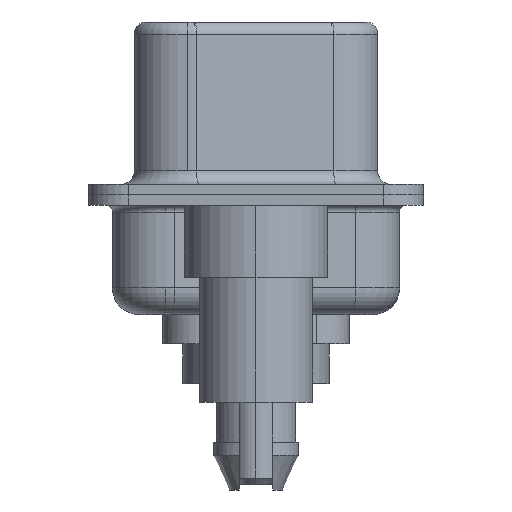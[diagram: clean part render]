
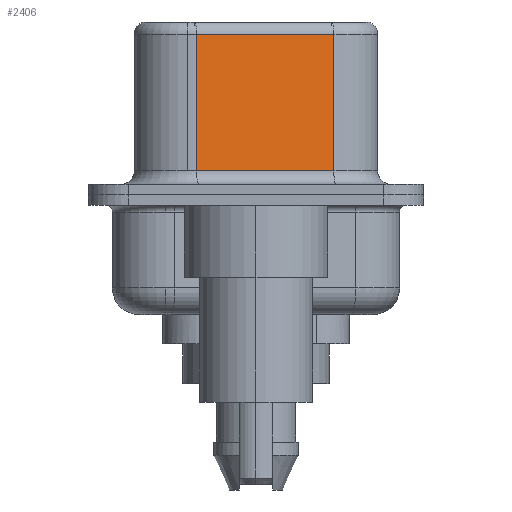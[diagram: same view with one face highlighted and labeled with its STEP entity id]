
A CAD part, left-side view. The second image highlights one B-rep face of the part: STEP entity #2406.
In plain terms, the highlighted planar face has unit normal (-0.985, -0.174, 0).
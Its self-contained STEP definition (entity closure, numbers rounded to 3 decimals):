
#32 = DIRECTION ( 'NONE',  ( 0., 0., -1. ) ) ;
#835 = CARTESIAN_POINT ( 'NONE',  ( 4.58, -2.927, 6.02 ) ) ;
#1250 = VERTEX_POINT ( 'NONE', #835 ) ;
#1404 = PLANE ( 'NONE',  #1975 ) ;
#1975 = AXIS2_PLACEMENT_3D ( 'NONE', #5075, #6692, #3466 ) ;
#2333 = ORIENTED_EDGE ( 'NONE', *, *, #19960, .F. ) ;
#2406 = ADVANCED_FACE ( 'NONE', ( #7004 ), #1404, .F. ) ;
#2916 = CARTESIAN_POINT ( 'NONE',  ( 3.67, 2.233, 0.9 ) ) ;
#2998 = DIRECTION ( 'NONE',  ( 0.174, -0.985, 0. ) ) ;
#3037 = LINE ( 'NONE', #17930, #7147 ) ;
#3466 = DIRECTION ( 'NONE',  ( -0.174, 0.985, 0. ) ) ;
#3701 = CARTESIAN_POINT ( 'NONE',  ( 4.58, -2.927, 6.52 ) ) ;
#4115 = ORIENTED_EDGE ( 'NONE', *, *, #10128, .T. ) ;
#4736 = LINE ( 'NONE', #3701, #11579 ) ;
#5075 = CARTESIAN_POINT ( 'NONE',  ( 4.58, -2.927, 6.52 ) ) ;
#6080 = LINE ( 'NONE', #13188, #12637 ) ;
#6348 = ORIENTED_EDGE ( 'NONE', *, *, #9032, .T. ) ;
#6692 = DIRECTION ( 'NONE',  ( 0.985, 0.174, 0. ) ) ;
#7004 = FACE_OUTER_BOUND ( 'NONE', #19315, .T. ) ;
#7147 = VECTOR ( 'NONE', #32, 1000. ) ;
#7214 = VERTEX_POINT ( 'NONE', #19812 ) ;
#7586 = ORIENTED_EDGE ( 'NONE', *, *, #13497, .T. ) ;
#9032 = EDGE_CURVE ( 'NONE', #20354, #9865, #3037, .T. ) ;
#9142 = DIRECTION ( 'NONE',  ( -0.174, 0.985, 0. ) ) ;
#9865 = VERTEX_POINT ( 'NONE', #2916 ) ;
#10128 = EDGE_CURVE ( 'NONE', #1250, #20354, #6080, .T. ) ;
#11579 = VECTOR ( 'NONE', #13399, 1000. ) ;
#12038 = LINE ( 'NONE', #20959, #19221 ) ;
#12637 = VECTOR ( 'NONE', #9142, 1000. ) ;
#13188 = CARTESIAN_POINT ( 'NONE',  ( 4.58, -2.927, 6.02 ) ) ;
#13399 = DIRECTION ( 'NONE',  ( 0., 0., -1. ) ) ;
#13497 = EDGE_CURVE ( 'NONE', #9865, #7214, #12038, .T. ) ;
#15834 = CARTESIAN_POINT ( 'NONE',  ( 3.67, 2.233, 6.02 ) ) ;
#17930 = CARTESIAN_POINT ( 'NONE',  ( 3.67, 2.233, 6.52 ) ) ;
#19221 = VECTOR ( 'NONE', #2998, 1000. ) ;
#19315 = EDGE_LOOP ( 'NONE', ( #2333, #4115, #6348, #7586 ) ) ;
#19812 = CARTESIAN_POINT ( 'NONE',  ( 4.58, -2.927, 0.9 ) ) ;
#19960 = EDGE_CURVE ( 'NONE', #1250, #7214, #4736, .T. ) ;
#20354 = VERTEX_POINT ( 'NONE', #15834 ) ;
#20959 = CARTESIAN_POINT ( 'NONE',  ( 4.58, -2.927, 0.9 ) ) ;
